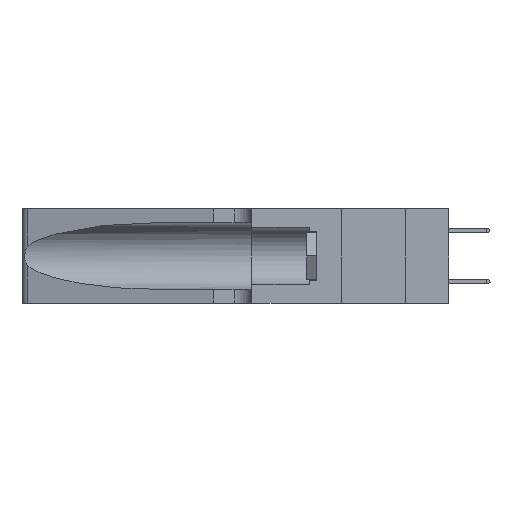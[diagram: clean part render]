
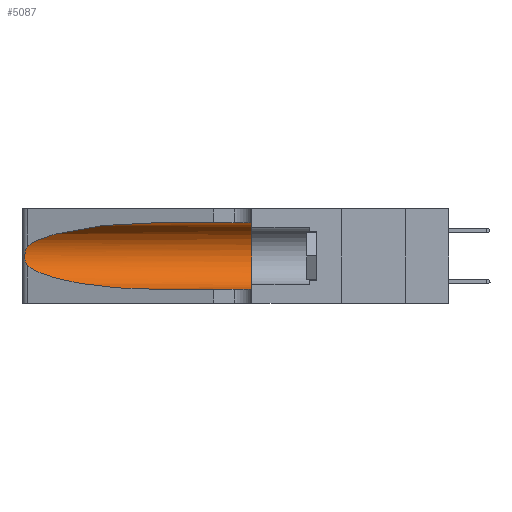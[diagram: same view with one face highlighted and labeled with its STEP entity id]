
A CAD part, left-side view. The second image highlights one B-rep face of the part: STEP entity #5087.
In plain terms, the highlighted cylindrical face has radius 3.308 mm (diameter 6.617 mm), a partial arc.
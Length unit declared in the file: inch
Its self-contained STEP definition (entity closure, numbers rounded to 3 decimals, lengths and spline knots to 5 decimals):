
#96 = EDGE_CURVE ( 'NONE', #32172, #29057, #36699, .T. ) ;
#694 = CARTESIAN_POINT ( 'NONE',  ( 0.1305, 0.72297, 0.05475 ) ) ;
#3293 = ORIENTED_EDGE ( 'NONE', *, *, #20205, .T. ) ;
#4027 = CARTESIAN_POINT ( 'NONE',  ( 0.25487, 1.22718, 0.22369 ) ) ;
#4334 = CYLINDRICAL_SURFACE ( 'NONE', #22542, 0.13025 ) ;
#4408 = VECTOR ( 'NONE', #8939, 39.37008 ) ;
#5087 = ADVANCED_FACE ( 'NONE', ( #32498 ), #4334, .F. ) ;
#5932 = CARTESIAN_POINT ( 'NONE',  ( 0.26075, 1.23896, 0.19203 ) ) ;
#6691 = CARTESIAN_POINT ( 'NONE',  ( 0.1305, 1.61858, 0.31525 ) ) ;
#7121 = CARTESIAN_POINT ( 'NONE',  ( 0.2373, 1.15595, 0.28018 ) ) ;
#7913 = CARTESIAN_POINT ( 'NONE',  ( 0.26018, 1.23835, 0.19895 ) ) ;
#8032 = EDGE_CURVE ( 'NONE', #29057, #16708, #13816, .T. ) ;
#8095 = VERTEX_POINT ( 'NONE', #18428 ) ;
#8534 = CARTESIAN_POINT ( 'NONE',  ( 0.25639, 1.23184, 0.21858 ) ) ;
#8864 = CARTESIAN_POINT ( 'NONE',  ( 0.25856, 1.23593, 0.16098 ) ) ;
#8939 = DIRECTION ( 'NONE',  ( 0., -1., 0. ) ) ;
#9039 = CARTESIAN_POINT ( 'NONE',  ( 0.1305, 1.61858, 0.05475 ) ) ;
#9484 = VECTOR ( 'NONE', #41938, 39.37008 ) ;
#9985 = CARTESIAN_POINT ( 'NONE',  ( 0.26075, 1.23896, 0.178 ) ) ;
#10746 = CARTESIAN_POINT ( 'NONE',  ( 0.25639, 1.23186, 0.15144 ) ) ;
#11116 = CARTESIAN_POINT ( 'NONE',  ( 0.1305, 0.35, 0.185 ) ) ;
#12495 = CARTESIAN_POINT ( 'NONE',  ( 0.25787, 1.23484, 0.2124 ) ) ;
#13816 = CIRCLE ( 'NONE', #15201, 0.13025 ) ;
#15106 = CARTESIAN_POINT ( 'NONE',  ( 0.1305, 0.35, 0.05475 ) ) ;
#15201 = AXIS2_PLACEMENT_3D ( 'NONE', #11116, #18598, #41724 ) ;
#15535 = ORIENTED_EDGE ( 'NONE', *, *, #96, .F. ) ;
#16074 = CARTESIAN_POINT ( 'NONE',  ( 0.1305, 0.72297, 0.05475 ) ) ;
#16179 = EDGE_CURVE ( 'NONE', #16355, #8095, #17243, .T. ) ;
#16355 = VERTEX_POINT ( 'NONE', #32376 ) ;
#16467 = CARTESIAN_POINT ( 'NONE',  ( 0.1305, 0.72297, 0.31525 ) ) ;
#16708 = VERTEX_POINT ( 'NONE', #15106 ) ;
#17102 = EDGE_LOOP ( 'NONE', ( #3293, #22966, #40783, #31723, #23100, #15535 ) ) ;
#17243 = B_SPLINE_CURVE_WITH_KNOTS ( 'NONE', 3,
 ( #4027, #23250, #8534, #12495, #29931, #7913, #5932, #9985, #40295, #8864, #27081, #10746, #23907, #28560 ),
 .UNSPECIFIED., .F., .F.,
 ( 4, 2, 2, 2, 2, 2, 4 ),
 ( 0., 0.00027, 0.00053, 0.00107, 0.0016, 0.00187, 0.00214 ),
 .UNSPECIFIED. ) ;
#17433 = CARTESIAN_POINT ( 'NONE',  ( 0.25487, 1.22718, 0.22369 ) ) ;
#18240 = LINE ( 'NONE', #9039, #9484 ) ;
#18428 = CARTESIAN_POINT ( 'NONE',  ( 0.25487, 1.22718, 0.14631 ) ) ;
#18573 =( BOUNDED_CURVE ( )  B_SPLINE_CURVE ( 3, ( #16467, #26324, #7121, #17433 ),
 .UNSPECIFIED., .F., .T. ) 
 B_SPLINE_CURVE_WITH_KNOTS ( ( 4, 4 ),
 ( 1.5708, 2.84003 ),
 .UNSPECIFIED. ) 
 CURVE ( )  GEOMETRIC_REPRESENTATION_ITEM ( )  RATIONAL_B_SPLINE_CURVE ( ( 1., 0.87, 0.87, 1. ) ) 
 REPRESENTATION_ITEM ( '' )  );
#18598 = DIRECTION ( 'NONE',  ( 0., 1., 0. ) ) ;
#19216 = CARTESIAN_POINT ( 'NONE',  ( 0.2373, 1.15595, 0.08982 ) ) ;
#20205 = EDGE_CURVE ( 'NONE', #32172, #16355, #18573, .T. ) ;
#21455 = DIRECTION ( 'NONE',  ( 0., -1., 0. ) ) ;
#21770 = EDGE_CURVE ( 'NONE', #41824, #16708, #18240, .T. ) ;
#22542 = AXIS2_PLACEMENT_3D ( 'NONE', #41145, #21455, #24720 ) ;
#22966 = ORIENTED_EDGE ( 'NONE', *, *, #16179, .T. ) ;
#23100 = ORIENTED_EDGE ( 'NONE', *, *, #8032, .F. ) ;
#23250 = CARTESIAN_POINT ( 'NONE',  ( 0.25555, 1.22994, 0.2215 ) ) ;
#23907 = CARTESIAN_POINT ( 'NONE',  ( 0.25555, 1.22993, 0.14849 ) ) ;
#24720 = DIRECTION ( 'NONE',  ( 0., 0., -1. ) ) ;
#26324 = CARTESIAN_POINT ( 'NONE',  ( 0.18966, 0.96281, 0.31525 ) ) ;
#27081 = CARTESIAN_POINT ( 'NONE',  ( 0.25789, 1.23486, 0.15765 ) ) ;
#28560 = CARTESIAN_POINT ( 'NONE',  ( 0.25487, 1.22718, 0.14631 ) ) ;
#29057 = VERTEX_POINT ( 'NONE', #32723 ) ;
#29931 = CARTESIAN_POINT ( 'NONE',  ( 0.25854, 1.2359, 0.20912 ) ) ;
#31723 = ORIENTED_EDGE ( 'NONE', *, *, #21770, .T. ) ;
#32172 = VERTEX_POINT ( 'NONE', #38067 ) ;
#32376 = CARTESIAN_POINT ( 'NONE',  ( 0.25487, 1.22718, 0.22369 ) ) ;
#32498 = FACE_OUTER_BOUND ( 'NONE', #17102, .T. ) ;
#32723 = CARTESIAN_POINT ( 'NONE',  ( 0.1305, 0.35, 0.31525 ) ) ;
#35691 = CARTESIAN_POINT ( 'NONE',  ( 0.25487, 1.22718, 0.14631 ) ) ;
#36261 = EDGE_CURVE ( 'NONE', #8095, #41824, #41728, .T. ) ;
#36699 = LINE ( 'NONE', #6691, #4408 ) ;
#38067 = CARTESIAN_POINT ( 'NONE',  ( 0.1305, 0.72297, 0.31525 ) ) ;
#40295 = CARTESIAN_POINT ( 'NONE',  ( 0.26017, 1.23833, 0.17102 ) ) ;
#40783 = ORIENTED_EDGE ( 'NONE', *, *, #36261, .T. ) ;
#41145 = CARTESIAN_POINT ( 'NONE',  ( 0.1305, 1.61858, 0.185 ) ) ;
#41724 = DIRECTION ( 'NONE',  ( 0., 0., 1. ) ) ;
#41728 =( BOUNDED_CURVE ( )  B_SPLINE_CURVE ( 3, ( #35691, #19216, #42061, #16074 ),
 .UNSPECIFIED., .F., .F. ) 
 B_SPLINE_CURVE_WITH_KNOTS ( ( 4, 4 ),
 ( 3.44316, 4.71239 ),
 .UNSPECIFIED. ) 
 CURVE ( )  GEOMETRIC_REPRESENTATION_ITEM ( )  RATIONAL_B_SPLINE_CURVE ( ( 1., 0.87, 0.87, 1. ) ) 
 REPRESENTATION_ITEM ( '' )  );
#41824 = VERTEX_POINT ( 'NONE', #694 ) ;
#41938 = DIRECTION ( 'NONE',  ( 0., -1., 0. ) ) ;
#42061 = CARTESIAN_POINT ( 'NONE',  ( 0.18966, 0.96281, 0.05475 ) ) ;
